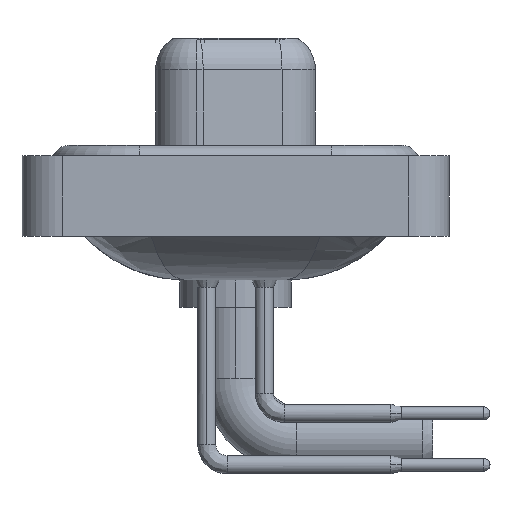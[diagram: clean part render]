
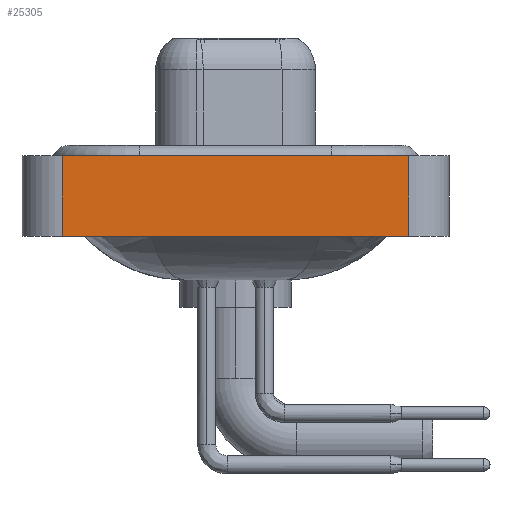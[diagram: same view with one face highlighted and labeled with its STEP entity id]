
A CAD part, left-side view. The second image highlights one B-rep face of the part: STEP entity #25305.
In plain terms, the highlighted planar face has unit normal (-1, 0, 0).
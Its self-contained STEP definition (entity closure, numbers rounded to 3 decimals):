
#666 = CARTESIAN_POINT ( 'NONE',  ( -7.35, -8.55, -3.6 ) ) ;
#1386 = DIRECTION ( 'NONE',  ( 0., -1., 0. ) ) ;
#2435 = EDGE_LOOP ( 'NONE', ( #17034, #23843, #18614, #10463 ) ) ;
#3186 = DIRECTION ( 'NONE',  ( -1., 0., 0. ) ) ;
#3828 = CARTESIAN_POINT ( 'NONE',  ( -7.35, -8.55, 0.4 ) ) ;
#4789 = VERTEX_POINT ( 'NONE', #3828 ) ;
#4928 = EDGE_CURVE ( 'NONE', #25715, #25857, #23608, .T. ) ;
#5300 = PLANE ( 'NONE',  #12573 ) ;
#5829 = DIRECTION ( 'NONE',  ( 0., -1., 0. ) ) ;
#6199 = DIRECTION ( 'NONE',  ( 0., 0., 1. ) ) ;
#6509 = VECTOR ( 'NONE', #1386, 1000. ) ;
#6595 = CARTESIAN_POINT ( 'NONE',  ( -7.35, -8.55, 0.4 ) ) ;
#7104 = CARTESIAN_POINT ( 'NONE',  ( -7.35, -8.55, -3.6 ) ) ;
#8358 = VECTOR ( 'NONE', #10903, 1000. ) ;
#9021 = FACE_OUTER_BOUND ( 'NONE', #2435, .T. ) ;
#10463 = ORIENTED_EDGE ( 'NONE', *, *, #4928, .T. ) ;
#10903 = DIRECTION ( 'NONE',  ( 0., 0., 1. ) ) ;
#11180 = VERTEX_POINT ( 'NONE', #24712 ) ;
#12267 = EDGE_CURVE ( 'NONE', #25857, #4789, #23155, .T. ) ;
#12573 = AXIS2_PLACEMENT_3D ( 'NONE', #16651, #3186, #17287 ) ;
#13649 = CARTESIAN_POINT ( 'NONE',  ( -7.35, 8.55, -3.6 ) ) ;
#16636 = EDGE_CURVE ( 'NONE', #11180, #4789, #25939, .T. ) ;
#16651 = CARTESIAN_POINT ( 'NONE',  ( -7.35, -8.55, -3.6 ) ) ;
#17034 = ORIENTED_EDGE ( 'NONE', *, *, #12267, .T. ) ;
#17287 = DIRECTION ( 'NONE',  ( 0., 0., 1. ) ) ;
#17471 = VECTOR ( 'NONE', #5829, 1000. ) ;
#18614 = ORIENTED_EDGE ( 'NONE', *, *, #20865, .F. ) ;
#20865 = EDGE_CURVE ( 'NONE', #25715, #11180, #24438, .T. ) ;
#22190 = CARTESIAN_POINT ( 'NONE',  ( -7.35, 8.55, -3.6 ) ) ;
#22840 = VECTOR ( 'NONE', #6199, 1000. ) ;
#23155 = LINE ( 'NONE', #666, #8358 ) ;
#23608 = LINE ( 'NONE', #7104, #6509 ) ;
#23843 = ORIENTED_EDGE ( 'NONE', *, *, #16636, .F. ) ;
#24438 = LINE ( 'NONE', #22190, #22840 ) ;
#24712 = CARTESIAN_POINT ( 'NONE',  ( -7.35, 8.55, 0.4 ) ) ;
#24958 = CARTESIAN_POINT ( 'NONE',  ( -7.35, -8.55, -3.6 ) ) ;
#25305 = ADVANCED_FACE ( 'NONE', ( #9021 ), #5300, .T. ) ;
#25715 = VERTEX_POINT ( 'NONE', #13649 ) ;
#25857 = VERTEX_POINT ( 'NONE', #24958 ) ;
#25939 = LINE ( 'NONE', #6595, #17471 ) ;
